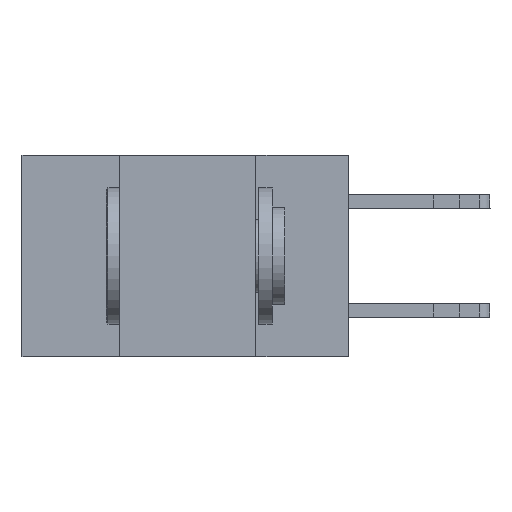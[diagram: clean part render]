
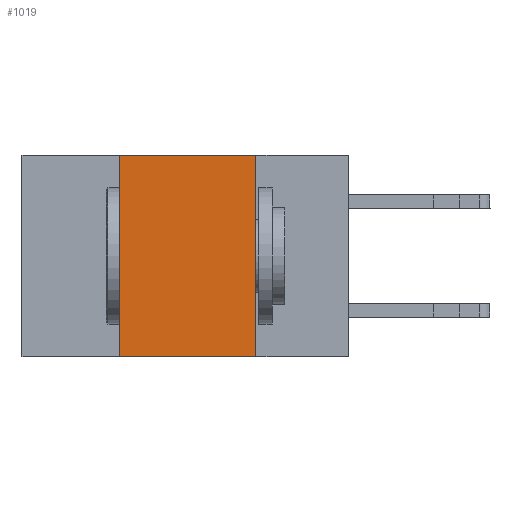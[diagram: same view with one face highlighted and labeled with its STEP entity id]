
A CAD part, left-side view. The second image highlights one B-rep face of the part: STEP entity #1019.
In plain terms, the highlighted planar face has unit normal (-1, 0, 0).
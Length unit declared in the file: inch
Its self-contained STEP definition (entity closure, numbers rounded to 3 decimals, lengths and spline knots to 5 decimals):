
#94 = CARTESIAN_POINT ( 'NONE',  ( 0., 0.6, 0. ) ) ;
#1019 = ADVANCED_FACE ( 'NONE', ( #1928 ), #15784, .F. ) ;
#1928 = FACE_OUTER_BOUND ( 'NONE', #18233, .T. ) ;
#2086 = VECTOR ( 'NONE', #20803, 39.37008 ) ;
#2154 = DIRECTION ( 'NONE',  ( 1., 0., 0. ) ) ;
#2930 = CARTESIAN_POINT ( 'NONE',  ( 0., 0.17, -0.37 ) ) ;
#3568 = LINE ( 'NONE', #17334, #13806 ) ;
#4213 = VERTEX_POINT ( 'NONE', #7071 ) ;
#4638 = DIRECTION ( 'NONE',  ( 0., 0., 1. ) ) ;
#5250 = CARTESIAN_POINT ( 'NONE',  ( 0., 0.17, -0.37 ) ) ;
#5539 = CARTESIAN_POINT ( 'NONE',  ( 0., 0.6, 0. ) ) ;
#5641 = VERTEX_POINT ( 'NONE', #2930 ) ;
#5658 = LINE ( 'NONE', #5539, #9211 ) ;
#7071 = CARTESIAN_POINT ( 'NONE',  ( 0., 0.42, 0. ) ) ;
#7488 = EDGE_CURVE ( 'NONE', #18973, #5641, #3568, .T. ) ;
#8700 = CARTESIAN_POINT ( 'NONE',  ( 0., 0.17, 0. ) ) ;
#9211 = VECTOR ( 'NONE', #16050, 39.37008 ) ;
#9581 = VECTOR ( 'NONE', #4638, 39.37008 ) ;
#9613 = EDGE_CURVE ( 'NONE', #18973, #4213, #21610, .T. ) ;
#11226 = EDGE_CURVE ( 'NONE', #4213, #12318, #5658, .T. ) ;
#12260 = CARTESIAN_POINT ( 'NONE',  ( 0., 0.42, -0.37 ) ) ;
#12318 = VERTEX_POINT ( 'NONE', #8700 ) ;
#12980 = ORIENTED_EDGE ( 'NONE', *, *, #11226, .F. ) ;
#13377 = ORIENTED_EDGE ( 'NONE', *, *, #16003, .F. ) ;
#13806 = VECTOR ( 'NONE', #15480, 39.37008 ) ;
#13921 = AXIS2_PLACEMENT_3D ( 'NONE', #94, #2154, #14060 ) ;
#14060 = DIRECTION ( 'NONE',  ( 0., 0., -1. ) ) ;
#14953 = ORIENTED_EDGE ( 'NONE', *, *, #7488, .T. ) ;
#15480 = DIRECTION ( 'NONE',  ( 0., -1., 0. ) ) ;
#15784 = PLANE ( 'NONE',  #13921 ) ;
#16003 = EDGE_CURVE ( 'NONE', #12318, #5641, #22517, .T. ) ;
#16050 = DIRECTION ( 'NONE',  ( 0., -1., 0. ) ) ;
#17334 = CARTESIAN_POINT ( 'NONE',  ( 0., 0.6, -0.37 ) ) ;
#18233 = EDGE_LOOP ( 'NONE', ( #13377, #12980, #22376, #14953 ) ) ;
#18973 = VERTEX_POINT ( 'NONE', #12260 ) ;
#20803 = DIRECTION ( 'NONE',  ( 0., 0., -1. ) ) ;
#21610 = LINE ( 'NONE', #22054, #9581 ) ;
#22054 = CARTESIAN_POINT ( 'NONE',  ( 0., 0.42, -0.37 ) ) ;
#22376 = ORIENTED_EDGE ( 'NONE', *, *, #9613, .F. ) ;
#22517 = LINE ( 'NONE', #5250, #2086 ) ;
